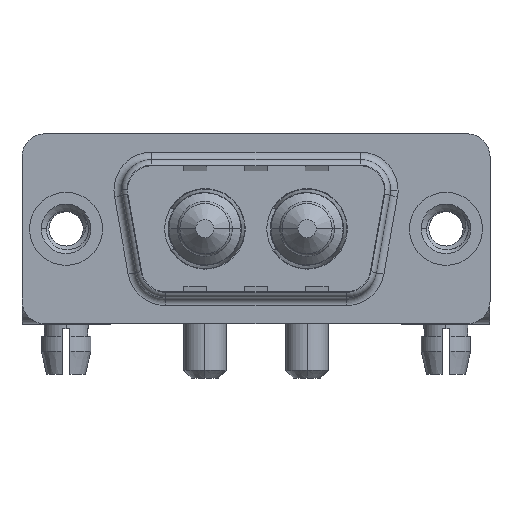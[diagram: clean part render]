
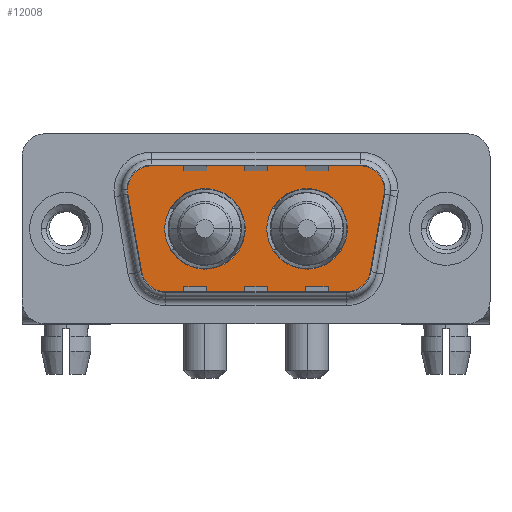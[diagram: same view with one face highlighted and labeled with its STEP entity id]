
A CAD part, top view. The second image highlights one B-rep face of the part: STEP entity #12008.
In plain terms, the highlighted planar face has unit normal (0, 0, 1).
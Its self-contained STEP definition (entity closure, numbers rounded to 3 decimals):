
#147 = CIRCLE ( 'NONE', #6308, 2. ) ;
#150 = FACE_BOUND ( 'NONE', #3334, .T. ) ;
#226 = DIRECTION ( 'NONE',  ( 0., 0., 1. ) ) ;
#538 = VERTEX_POINT ( 'NONE', #3040 ) ;
#621 = AXIS2_PLACEMENT_3D ( 'NONE', #1646, #12521, #11372 ) ;
#688 = ORIENTED_EDGE ( 'NONE', *, *, #9853, .F. ) ;
#710 = EDGE_CURVE ( 'NONE', #11535, #2847, #13239, .T. ) ;
#864 = DIRECTION ( 'NONE',  ( 0., 0., 1. ) ) ;
#928 = ORIENTED_EDGE ( 'NONE', *, *, #13932, .F. ) ;
#976 = VERTEX_POINT ( 'NONE', #5289 ) ;
#1010 = DIRECTION ( 'NONE',  ( 1., 0., 0. ) ) ;
#1250 = CARTESIAN_POINT ( 'NONE',  ( 20.511, -3.247, 0. ) ) ;
#1314 = ORIENTED_EDGE ( 'NONE', *, *, #11208, .T. ) ;
#1315 = LINE ( 'NONE', #6786, #5507 ) ;
#1434 = EDGE_CURVE ( 'NONE', #2847, #2620, #1724, .T. ) ;
#1540 = ORIENTED_EDGE ( 'NONE', *, *, #5443, .T. ) ;
#1541 = ORIENTED_EDGE ( 'NONE', *, *, #1648, .F. ) ;
#1577 = ORIENTED_EDGE ( 'NONE', *, *, #13464, .T. ) ;
#1646 = CARTESIAN_POINT ( 'NONE',  ( 9.14, 0., 0. ) ) ;
#1648 = EDGE_CURVE ( 'NONE', #8793, #3982, #4668, .T. ) ;
#1688 = DIRECTION ( 'NONE',  ( 1., 0., 0. ) ) ;
#1724 = CIRCLE ( 'NONE', #11762, 2. ) ;
#1938 = CARTESIAN_POINT ( 'NONE',  ( 13.21, 0., 0. ) ) ;
#2274 = ORIENTED_EDGE ( 'NONE', *, *, #1434, .T. ) ;
#2294 = DIRECTION ( 'NONE',  ( 0., 0., 1. ) ) ;
#2307 = CARTESIAN_POINT ( 'NONE',  ( 5.436, 4.9, 0. ) ) ;
#2571 = VERTEX_POINT ( 'NONE', #2307 ) ;
#2620 = VERTEX_POINT ( 'NONE', #3594 ) ;
#2751 = CARTESIAN_POINT ( 'NONE',  ( 19.564, 4.9, 0. ) ) ;
#2847 = VERTEX_POINT ( 'NONE', #11797 ) ;
#2883 = CARTESIAN_POINT ( 'NONE',  ( 6.459, -4.9, 0. ) ) ;
#2971 = DIRECTION ( 'NONE',  ( 0., 0., 1. ) ) ;
#3040 = CARTESIAN_POINT ( 'NONE',  ( 18.541, -4.9, 0. ) ) ;
#3224 = ORIENTED_EDGE ( 'NONE', *, *, #13310, .T. ) ;
#3319 = DIRECTION ( 'NONE',  ( 0.174, -0.985, 0. ) ) ;
#3334 = EDGE_LOOP ( 'NONE', ( #928, #1541 ) ) ;
#3389 = DIRECTION ( 'NONE',  ( 0., 0., 1. ) ) ;
#3594 = CARTESIAN_POINT ( 'NONE',  ( 21.564, 2.9, 0. ) ) ;
#3982 = VERTEX_POINT ( 'NONE', #9873 ) ;
#4196 = DIRECTION ( 'NONE',  ( 1., 0., 0. ) ) ;
#4382 = CARTESIAN_POINT ( 'NONE',  ( 6.459, -2.9, 0. ) ) ;
#4454 = DIRECTION ( 'NONE',  ( 0.174, 0.985, 0. ) ) ;
#4668 = CIRCLE ( 'NONE', #10392, 2.65 ) ;
#4823 = CARTESIAN_POINT ( 'NONE',  ( 15.86, 0., 0. ) ) ;
#5205 = EDGE_LOOP ( 'NONE', ( #7026, #688 ) ) ;
#5256 = VERTEX_POINT ( 'NONE', #6030 ) ;
#5289 = CARTESIAN_POINT ( 'NONE',  ( 3.466, 2.553, 0. ) ) ;
#5424 = DIRECTION ( 'NONE',  ( 1., 0., 0. ) ) ;
#5443 = EDGE_CURVE ( 'NONE', #976, #5256, #1315, .T. ) ;
#5507 = VECTOR ( 'NONE', #3319, 1000. ) ;
#5517 = CARTESIAN_POINT ( 'NONE',  ( 21.534, 2.553, 0. ) ) ;
#5570 = CIRCLE ( 'NONE', #12886, 2.65 ) ;
#5724 = FACE_OUTER_BOUND ( 'NONE', #11677, .T. ) ;
#5726 = CARTESIAN_POINT ( 'NONE',  ( 18.541, -2.9, 0. ) ) ;
#5844 = CARTESIAN_POINT ( 'NONE',  ( 5.436, 4.9, 0. ) ) ;
#5852 = VERTEX_POINT ( 'NONE', #2883 ) ;
#5926 = LINE ( 'NONE', #5844, #9558 ) ;
#6030 = CARTESIAN_POINT ( 'NONE',  ( 4.489, -3.247, 0. ) ) ;
#6308 = AXIS2_PLACEMENT_3D ( 'NONE', #4382, #3389, #11092 ) ;
#6320 = DIRECTION ( 'NONE',  ( 0., 0., 1. ) ) ;
#6514 = CARTESIAN_POINT ( 'NONE',  ( 6.49, 0., 0. ) ) ;
#6534 = AXIS2_PLACEMENT_3D ( 'NONE', #10026, #8878, #13229 ) ;
#6695 = VECTOR ( 'NONE', #4454, 1000. ) ;
#6786 = CARTESIAN_POINT ( 'NONE',  ( 3.466, 2.553, 0. ) ) ;
#7026 = ORIENTED_EDGE ( 'NONE', *, *, #8928, .F. ) ;
#7571 = PLANE ( 'NONE',  #6534 ) ;
#7620 = EDGE_CURVE ( 'NONE', #13575, #2571, #5926, .T. ) ;
#7849 = FACE_BOUND ( 'NONE', #5205, .T. ) ;
#8143 = AXIS2_PLACEMENT_3D ( 'NONE', #5726, #226, #11011 ) ;
#8419 = ORIENTED_EDGE ( 'NONE', *, *, #12395, .T. ) ;
#8526 = CIRCLE ( 'NONE', #9894, 2.65 ) ;
#8715 = CARTESIAN_POINT ( 'NONE',  ( 9.14, 0., 0. ) ) ;
#8743 = CARTESIAN_POINT ( 'NONE',  ( 15.86, 0., 0. ) ) ;
#8793 = VERTEX_POINT ( 'NONE', #6514 ) ;
#8824 = CIRCLE ( 'NONE', #12493, 2. ) ;
#8878 = DIRECTION ( 'NONE',  ( 0., 0., 1. ) ) ;
#8928 = EDGE_CURVE ( 'NONE', #13816, #13825, #8526, .T. ) ;
#9077 = VECTOR ( 'NONE', #1010, 1000. ) ;
#9233 = ORIENTED_EDGE ( 'NONE', *, *, #13414, .T. ) ;
#9525 = DIRECTION ( 'NONE',  ( -1., 0., 0. ) ) ;
#9558 = VECTOR ( 'NONE', #13209, 1000. ) ;
#9683 = DIRECTION ( 'NONE',  ( 1., 0., 0. ) ) ;
#9719 = LINE ( 'NONE', #12223, #9077 ) ;
#9853 = EDGE_CURVE ( 'NONE', #13825, #13816, #5570, .T. ) ;
#9873 = CARTESIAN_POINT ( 'NONE',  ( 11.79, 0., 0. ) ) ;
#9894 = AXIS2_PLACEMENT_3D ( 'NONE', #8743, #6320, #9683 ) ;
#10026 = CARTESIAN_POINT ( 'NONE',  ( 18.541, -2.9, 0. ) ) ;
#10392 = AXIS2_PLACEMENT_3D ( 'NONE', #8715, #2294, #5424 ) ;
#10410 = AXIS2_PLACEMENT_3D ( 'NONE', #13262, #13481, #1688 ) ;
#10441 = DIRECTION ( 'NONE',  ( -1., 0., 0. ) ) ;
#10511 = CARTESIAN_POINT ( 'NONE',  ( 19.564, 2.9, 0. ) ) ;
#11011 = DIRECTION ( 'NONE',  ( 1., 0., 0. ) ) ;
#11091 = CIRCLE ( 'NONE', #10410, 2. ) ;
#11092 = DIRECTION ( 'NONE',  ( -1., 0., 0. ) ) ;
#11208 = EDGE_CURVE ( 'NONE', #2571, #976, #11091, .T. ) ;
#11353 = CIRCLE ( 'NONE', #8143, 2. ) ;
#11372 = DIRECTION ( 'NONE',  ( 1., 0., 0. ) ) ;
#11535 = VERTEX_POINT ( 'NONE', #1250 ) ;
#11614 = DIRECTION ( 'NONE',  ( 0., 0., 1. ) ) ;
#11677 = EDGE_LOOP ( 'NONE', ( #1577, #12253, #2274, #3224, #12240, #1314, #1540, #9233, #8419 ) ) ;
#11762 = AXIS2_PLACEMENT_3D ( 'NONE', #10511, #864, #10441 ) ;
#11797 = CARTESIAN_POINT ( 'NONE',  ( 21.534, 2.553, 0. ) ) ;
#12008 = ADVANCED_FACE ( 'NONE', ( #7849, #150, #5724 ), #7571, .T. ) ;
#12223 = CARTESIAN_POINT ( 'NONE',  ( 6.459, -4.9, 0. ) ) ;
#12240 = ORIENTED_EDGE ( 'NONE', *, *, #7620, .T. ) ;
#12253 = ORIENTED_EDGE ( 'NONE', *, *, #710, .T. ) ;
#12395 = EDGE_CURVE ( 'NONE', #5852, #538, #9719, .T. ) ;
#12493 = AXIS2_PLACEMENT_3D ( 'NONE', #12758, #2971, #9525 ) ;
#12521 = DIRECTION ( 'NONE',  ( 0., 0., 1. ) ) ;
#12736 = CIRCLE ( 'NONE', #621, 2.65 ) ;
#12758 = CARTESIAN_POINT ( 'NONE',  ( 19.564, 2.9, 0. ) ) ;
#12886 = AXIS2_PLACEMENT_3D ( 'NONE', #4823, #11614, #4196 ) ;
#13209 = DIRECTION ( 'NONE',  ( -1., 0., 0. ) ) ;
#13229 = DIRECTION ( 'NONE',  ( 1., 0., 0. ) ) ;
#13239 = LINE ( 'NONE', #5517, #6695 ) ;
#13262 = CARTESIAN_POINT ( 'NONE',  ( 5.436, 2.9, 0. ) ) ;
#13310 = EDGE_CURVE ( 'NONE', #2620, #13575, #8824, .T. ) ;
#13414 = EDGE_CURVE ( 'NONE', #5256, #5852, #147, .T. ) ;
#13464 = EDGE_CURVE ( 'NONE', #538, #11535, #11353, .T. ) ;
#13481 = DIRECTION ( 'NONE',  ( 0., 0., 1. ) ) ;
#13575 = VERTEX_POINT ( 'NONE', #2751 ) ;
#13816 = VERTEX_POINT ( 'NONE', #13871 ) ;
#13825 = VERTEX_POINT ( 'NONE', #1938 ) ;
#13871 = CARTESIAN_POINT ( 'NONE',  ( 18.51, 0., 0. ) ) ;
#13932 = EDGE_CURVE ( 'NONE', #3982, #8793, #12736, .T. ) ;
